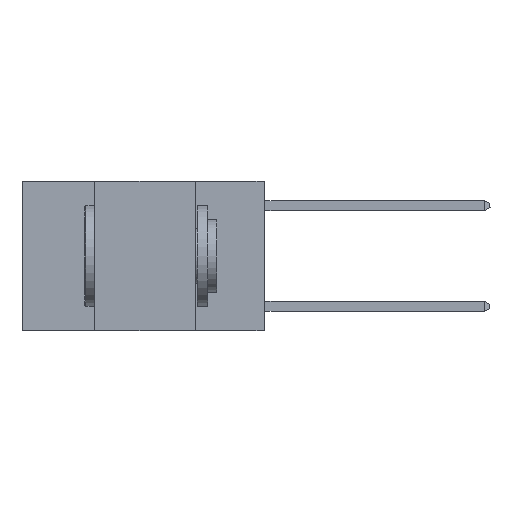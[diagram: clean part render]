
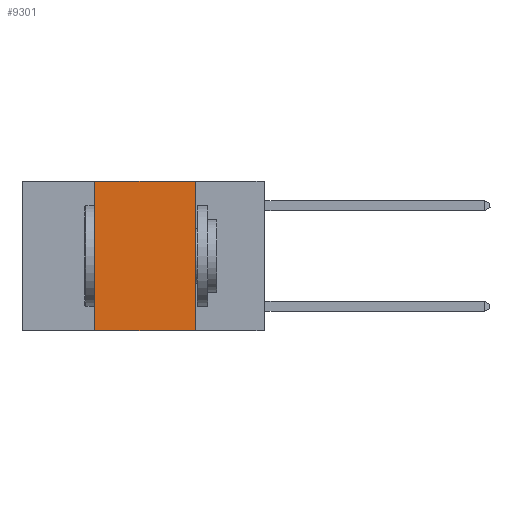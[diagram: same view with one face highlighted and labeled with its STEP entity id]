
A CAD part, left-side view. The second image highlights one B-rep face of the part: STEP entity #9301.
In plain terms, the highlighted planar face has unit normal (-1, 0, 0).
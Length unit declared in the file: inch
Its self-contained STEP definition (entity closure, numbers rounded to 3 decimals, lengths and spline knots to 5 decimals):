
#1678 = EDGE_LOOP ( 'NONE', ( #10363, #15673, #7940, #8085 ) ) ;
#2346 = EDGE_CURVE ( 'NONE', #6483, #2824, #6969, .T. ) ;
#2356 = CARTESIAN_POINT ( 'NONE',  ( 0., 0.6, 0. ) ) ;
#2699 = VECTOR ( 'NONE', #10304, 39.37008 ) ;
#2824 = VERTEX_POINT ( 'NONE', #12865 ) ;
#3545 = DIRECTION ( 'NONE',  ( 1., 0., 0. ) ) ;
#4257 = DIRECTION ( 'NONE',  ( 0., 0., 1. ) ) ;
#4492 = VECTOR ( 'NONE', #11159, 39.37008 ) ;
#4591 = LINE ( 'NONE', #10497, #7467 ) ;
#4699 = CARTESIAN_POINT ( 'NONE',  ( 0., 0.42, 0. ) ) ;
#4714 = CARTESIAN_POINT ( 'NONE',  ( 0., 0.17, -0.37 ) ) ;
#6483 = VERTEX_POINT ( 'NONE', #4699 ) ;
#6969 = LINE ( 'NONE', #10073, #7532 ) ;
#7351 = LINE ( 'NONE', #9958, #4492 ) ;
#7467 = VECTOR ( 'NONE', #4257, 39.37008 ) ;
#7532 = VECTOR ( 'NONE', #9952, 39.37008 ) ;
#7940 = ORIENTED_EDGE ( 'NONE', *, *, #8586, .F. ) ;
#8085 = ORIENTED_EDGE ( 'NONE', *, *, #10947, .T. ) ;
#8516 = EDGE_CURVE ( 'NONE', #2824, #15309, #12609, .T. ) ;
#8586 = EDGE_CURVE ( 'NONE', #9395, #6483, #4591, .T. ) ;
#8698 = CARTESIAN_POINT ( 'NONE',  ( 0., 0.42, -0.37 ) ) ;
#8988 = CARTESIAN_POINT ( 'NONE',  ( 0., 0.17, 0. ) ) ;
#9301 = ADVANCED_FACE ( 'NONE', ( #14076 ), #9733, .F. ) ;
#9395 = VERTEX_POINT ( 'NONE', #8698 ) ;
#9733 = PLANE ( 'NONE',  #13246 ) ;
#9952 = DIRECTION ( 'NONE',  ( 0., -1., 0. ) ) ;
#9958 = CARTESIAN_POINT ( 'NONE',  ( 0., 0.6, -0.37 ) ) ;
#10073 = CARTESIAN_POINT ( 'NONE',  ( 0., 0.6, 0. ) ) ;
#10304 = DIRECTION ( 'NONE',  ( 0., 0., -1. ) ) ;
#10363 = ORIENTED_EDGE ( 'NONE', *, *, #8516, .F. ) ;
#10497 = CARTESIAN_POINT ( 'NONE',  ( 0., 0.42, 0. ) ) ;
#10947 = EDGE_CURVE ( 'NONE', #9395, #15309, #7351, .T. ) ;
#11159 = DIRECTION ( 'NONE',  ( 0., -1., 0. ) ) ;
#12292 = DIRECTION ( 'NONE',  ( 0., 0., -1. ) ) ;
#12609 = LINE ( 'NONE', #8988, #2699 ) ;
#12865 = CARTESIAN_POINT ( 'NONE',  ( 0., 0.17, 0. ) ) ;
#13246 = AXIS2_PLACEMENT_3D ( 'NONE', #2356, #3545, #12292 ) ;
#14076 = FACE_OUTER_BOUND ( 'NONE', #1678, .T. ) ;
#15309 = VERTEX_POINT ( 'NONE', #4714 ) ;
#15673 = ORIENTED_EDGE ( 'NONE', *, *, #2346, .F. ) ;
